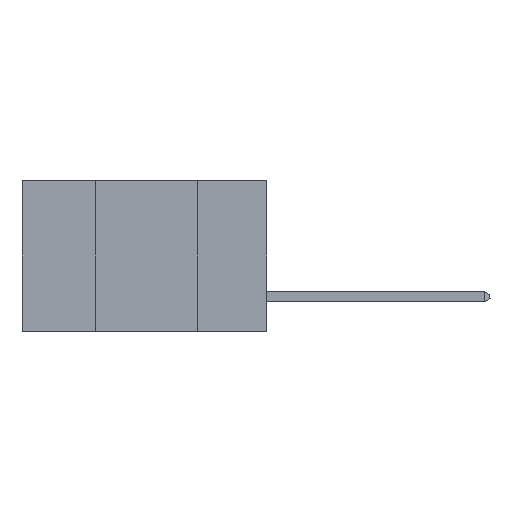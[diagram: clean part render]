
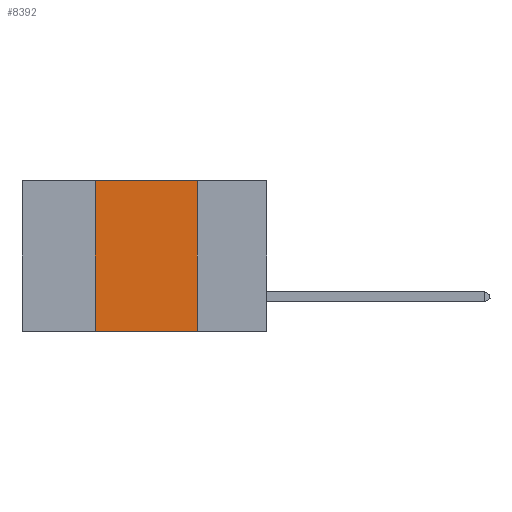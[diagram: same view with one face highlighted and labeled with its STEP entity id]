
A CAD part, left-side view. The second image highlights one B-rep face of the part: STEP entity #8392.
In plain terms, the highlighted planar face has unit normal (-1, 0, 0).
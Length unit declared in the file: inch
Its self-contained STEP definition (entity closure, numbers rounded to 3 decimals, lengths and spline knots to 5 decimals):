
#2611 = VERTEX_POINT ( 'NONE', #26081 ) ;
#3680 = DIRECTION ( 'NONE',  ( 0., -1., 0. ) ) ;
#4594 = VECTOR ( 'NONE', #26418, 39.37008 ) ;
#4865 = ORIENTED_EDGE ( 'NONE', *, *, #13085, .F. ) ;
#5497 = EDGE_CURVE ( 'NONE', #17166, #2611, #12408, .T. ) ;
#6661 = CARTESIAN_POINT ( 'NONE',  ( 0., 0.6, 0. ) ) ;
#7564 = CARTESIAN_POINT ( 'NONE',  ( 0., 0.6, -0.37 ) ) ;
#8392 = ADVANCED_FACE ( 'NONE', ( #42263 ), #17194, .F. ) ;
#8439 = LINE ( 'NONE', #43845, #4594 ) ;
#9862 = CARTESIAN_POINT ( 'NONE',  ( 0., 0.6, 0. ) ) ;
#10766 = EDGE_LOOP ( 'NONE', ( #19590, #4865, #12124, #29989 ) ) ;
#11118 = LINE ( 'NONE', #16818, #32436 ) ;
#11524 = VERTEX_POINT ( 'NONE', #42271 ) ;
#12124 = ORIENTED_EDGE ( 'NONE', *, *, #38011, .F. ) ;
#12408 = LINE ( 'NONE', #7564, #41955 ) ;
#12967 = DIRECTION ( 'NONE',  ( 0., 0., -1. ) ) ;
#13085 = EDGE_CURVE ( 'NONE', #36841, #11524, #29848, .T. ) ;
#16818 = CARTESIAN_POINT ( 'NONE',  ( 0., 0.17, 0. ) ) ;
#17166 = VERTEX_POINT ( 'NONE', #43626 ) ;
#17194 = PLANE ( 'NONE',  #21735 ) ;
#19590 = ORIENTED_EDGE ( 'NONE', *, *, #22173, .F. ) ;
#21735 = AXIS2_PLACEMENT_3D ( 'NONE', #9862, #45160, #41784 ) ;
#22173 = EDGE_CURVE ( 'NONE', #11524, #2611, #11118, .T. ) ;
#26081 = CARTESIAN_POINT ( 'NONE',  ( 0., 0.17, -0.37 ) ) ;
#26418 = DIRECTION ( 'NONE',  ( 0., 0., 1. ) ) ;
#29848 = LINE ( 'NONE', #6661, #31475 ) ;
#29989 = ORIENTED_EDGE ( 'NONE', *, *, #5497, .T. ) ;
#31475 = VECTOR ( 'NONE', #34357, 39.37008 ) ;
#32436 = VECTOR ( 'NONE', #12967, 39.37008 ) ;
#34357 = DIRECTION ( 'NONE',  ( 0., -1., 0. ) ) ;
#36841 = VERTEX_POINT ( 'NONE', #40733 ) ;
#38011 = EDGE_CURVE ( 'NONE', #17166, #36841, #8439, .T. ) ;
#40733 = CARTESIAN_POINT ( 'NONE',  ( 0., 0.42, 0. ) ) ;
#41784 = DIRECTION ( 'NONE',  ( 0., 0., -1. ) ) ;
#41955 = VECTOR ( 'NONE', #3680, 39.37008 ) ;
#42263 = FACE_OUTER_BOUND ( 'NONE', #10766, .T. ) ;
#42271 = CARTESIAN_POINT ( 'NONE',  ( 0., 0.17, 0. ) ) ;
#43626 = CARTESIAN_POINT ( 'NONE',  ( 0., 0.42, -0.37 ) ) ;
#43845 = CARTESIAN_POINT ( 'NONE',  ( 0., 0.42, 0. ) ) ;
#45160 = DIRECTION ( 'NONE',  ( 1., 0., 0. ) ) ;
